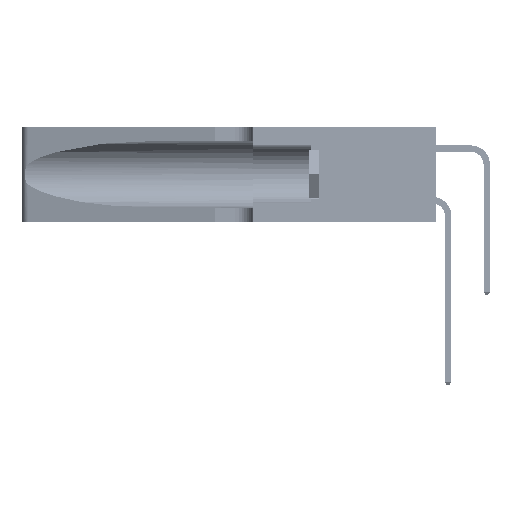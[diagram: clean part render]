
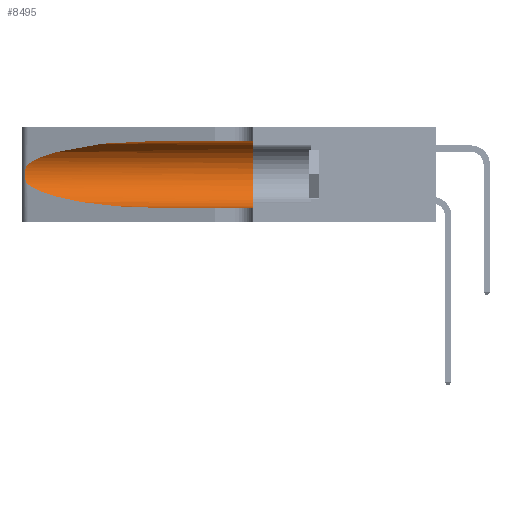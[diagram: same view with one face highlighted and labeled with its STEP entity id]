
A CAD part, left-side view. The second image highlights one B-rep face of the part: STEP entity #8495.
In plain terms, the highlighted cylindrical face has radius 3.308 mm (diameter 6.617 mm), a partial arc.
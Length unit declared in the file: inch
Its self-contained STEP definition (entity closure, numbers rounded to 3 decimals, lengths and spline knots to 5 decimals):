
#243 = EDGE_CURVE ( 'NONE', #27568, #1937, #8975, .T. ) ;
#575 = DIRECTION ( 'NONE',  ( 0., 1., 0. ) ) ;
#1230 = CARTESIAN_POINT ( 'NONE',  ( 0.25487, 1.22718, 0.14631 ) ) ;
#1275 = CARTESIAN_POINT ( 'NONE',  ( 0.26018, 1.23835, 0.19895 ) ) ;
#1579 = DIRECTION ( 'NONE',  ( 0., -1., 0. ) ) ;
#1937 = VERTEX_POINT ( 'NONE', #19312 ) ;
#4107 = EDGE_CURVE ( 'NONE', #7412, #6198, #24047, .T. ) ;
#5278 = CARTESIAN_POINT ( 'NONE',  ( 0.2373, 1.15595, 0.08982 ) ) ;
#5326 = CARTESIAN_POINT ( 'NONE',  ( 0.26075, 1.23896, 0.178 ) ) ;
#5626 = DIRECTION ( 'NONE',  ( 0., 0., -1. ) ) ;
#6198 = VERTEX_POINT ( 'NONE', #50195 ) ;
#6496 = EDGE_LOOP ( 'NONE', ( #50033, #46082, #17295, #17205, #7360, #41811 ) ) ;
#7360 = ORIENTED_EDGE ( 'NONE', *, *, #22067, .F. ) ;
#7412 = VERTEX_POINT ( 'NONE', #39130 ) ;
#8495 = ADVANCED_FACE ( 'NONE', ( #29424 ), #28203, .F. ) ;
#8975 =( BOUNDED_CURVE ( )  B_SPLINE_CURVE ( 3, ( #45975, #42132, #22733, #49862 ),
 .UNSPECIFIED., .F., .T. ) 
 B_SPLINE_CURVE_WITH_KNOTS ( ( 4, 4 ),
 ( 1.5708, 2.84003 ),
 .UNSPECIFIED. ) 
 CURVE ( )  GEOMETRIC_REPRESENTATION_ITEM ( )  RATIONAL_B_SPLINE_CURVE ( ( 1., 0.87, 0.87, 1. ) ) 
 REPRESENTATION_ITEM ( '' )  );
#9319 = CARTESIAN_POINT ( 'NONE',  ( 0.1305, 0.72297, 0.05475 ) ) ;
#9369 = CARTESIAN_POINT ( 'NONE',  ( 0.25856, 1.23593, 0.16098 ) ) ;
#10896 = VERTEX_POINT ( 'NONE', #24713 ) ;
#12718 = AXIS2_PLACEMENT_3D ( 'NONE', #24147, #575, #28016 ) ;
#13281 = CARTESIAN_POINT ( 'NONE',  ( 0.25639, 1.23186, 0.15144 ) ) ;
#14935 = CARTESIAN_POINT ( 'NONE',  ( 0.1305, 1.61858, 0.31525 ) ) ;
#17163 = CARTESIAN_POINT ( 'NONE',  ( 0.25487, 1.22718, 0.14631 ) ) ;
#17205 = ORIENTED_EDGE ( 'NONE', *, *, #4107, .T. ) ;
#17295 = ORIENTED_EDGE ( 'NONE', *, *, #40828, .T. ) ;
#19312 = CARTESIAN_POINT ( 'NONE',  ( 0.25487, 1.22718, 0.22369 ) ) ;
#19588 = B_SPLINE_CURVE_WITH_KNOTS ( 'NONE', 3,
 ( #40303, #44173, #20939, #48054, #24803, #1275, #28687, #5326, #32610, #9369, #36507, #13281, #40468, #17163 ),
 .UNSPECIFIED., .F., .F.,
 ( 4, 2, 2, 2, 2, 2, 4 ),
 ( 0., 0.00027, 0.00053, 0.00107, 0.0016, 0.00187, 0.00214 ),
 .UNSPECIFIED. ) ;
#20324 = CARTESIAN_POINT ( 'NONE',  ( 0.1305, 1.61858, 0.05475 ) ) ;
#20939 = CARTESIAN_POINT ( 'NONE',  ( 0.25639, 1.23184, 0.21858 ) ) ;
#21217 = CARTESIAN_POINT ( 'NONE',  ( 0.1305, 1.61858, 0.185 ) ) ;
#22067 = EDGE_CURVE ( 'NONE', #10896, #6198, #35866, .T. ) ;
#22733 = CARTESIAN_POINT ( 'NONE',  ( 0.2373, 1.15595, 0.28018 ) ) ;
#24047 = LINE ( 'NONE', #20324, #33134 ) ;
#24147 = CARTESIAN_POINT ( 'NONE',  ( 0.1305, 0.35, 0.185 ) ) ;
#24713 = CARTESIAN_POINT ( 'NONE',  ( 0.1305, 0.35, 0.31525 ) ) ;
#24803 = CARTESIAN_POINT ( 'NONE',  ( 0.25854, 1.2359, 0.20912 ) ) ;
#27568 = VERTEX_POINT ( 'NONE', #48504 ) ;
#28016 = DIRECTION ( 'NONE',  ( 0., 0., 1. ) ) ;
#28203 = CYLINDRICAL_SURFACE ( 'NONE', #32509, 0.13025 ) ;
#28687 = CARTESIAN_POINT ( 'NONE',  ( 0.26075, 1.23896, 0.19203 ) ) ;
#28864 = EDGE_CURVE ( 'NONE', #1937, #29435, #19588, .T. ) ;
#29385 = VECTOR ( 'NONE', #34627, 39.37008 ) ;
#29424 = FACE_OUTER_BOUND ( 'NONE', #6496, .T. ) ;
#29435 = VERTEX_POINT ( 'NONE', #50085 ) ;
#30047 = EDGE_CURVE ( 'NONE', #27568, #10896, #30609, .T. ) ;
#30609 = LINE ( 'NONE', #14935, #29385 ) ;
#32509 = AXIS2_PLACEMENT_3D ( 'NONE', #21217, #1579, #5626 ) ;
#32563 = CARTESIAN_POINT ( 'NONE',  ( 0.18966, 0.96281, 0.05475 ) ) ;
#32610 = CARTESIAN_POINT ( 'NONE',  ( 0.26017, 1.23833, 0.17102 ) ) ;
#33134 = VECTOR ( 'NONE', #43573, 39.37008 ) ;
#34627 = DIRECTION ( 'NONE',  ( 0., -1., 0. ) ) ;
#35866 = CIRCLE ( 'NONE', #12718, 0.13025 ) ;
#36507 = CARTESIAN_POINT ( 'NONE',  ( 0.25789, 1.23486, 0.15765 ) ) ;
#39130 = CARTESIAN_POINT ( 'NONE',  ( 0.1305, 0.72297, 0.05475 ) ) ;
#40303 = CARTESIAN_POINT ( 'NONE',  ( 0.25487, 1.22718, 0.22369 ) ) ;
#40468 = CARTESIAN_POINT ( 'NONE',  ( 0.25555, 1.22993, 0.14849 ) ) ;
#40828 = EDGE_CURVE ( 'NONE', #29435, #7412, #42943, .T. ) ;
#41811 = ORIENTED_EDGE ( 'NONE', *, *, #30047, .F. ) ;
#42132 = CARTESIAN_POINT ( 'NONE',  ( 0.18966, 0.96281, 0.31525 ) ) ;
#42943 =( BOUNDED_CURVE ( )  B_SPLINE_CURVE ( 3, ( #1230, #5278, #32563, #9319 ),
 .UNSPECIFIED., .F., .F. ) 
 B_SPLINE_CURVE_WITH_KNOTS ( ( 4, 4 ),
 ( 3.44316, 4.71239 ),
 .UNSPECIFIED. ) 
 CURVE ( )  GEOMETRIC_REPRESENTATION_ITEM ( )  RATIONAL_B_SPLINE_CURVE ( ( 1., 0.87, 0.87, 1. ) ) 
 REPRESENTATION_ITEM ( '' )  );
#43573 = DIRECTION ( 'NONE',  ( 0., -1., 0. ) ) ;
#44173 = CARTESIAN_POINT ( 'NONE',  ( 0.25555, 1.22994, 0.2215 ) ) ;
#45975 = CARTESIAN_POINT ( 'NONE',  ( 0.1305, 0.72297, 0.31525 ) ) ;
#46082 = ORIENTED_EDGE ( 'NONE', *, *, #28864, .T. ) ;
#48054 = CARTESIAN_POINT ( 'NONE',  ( 0.25787, 1.23484, 0.2124 ) ) ;
#48504 = CARTESIAN_POINT ( 'NONE',  ( 0.1305, 0.72297, 0.31525 ) ) ;
#49862 = CARTESIAN_POINT ( 'NONE',  ( 0.25487, 1.22718, 0.22369 ) ) ;
#50033 = ORIENTED_EDGE ( 'NONE', *, *, #243, .T. ) ;
#50085 = CARTESIAN_POINT ( 'NONE',  ( 0.25487, 1.22718, 0.14631 ) ) ;
#50195 = CARTESIAN_POINT ( 'NONE',  ( 0.1305, 0.35, 0.05475 ) ) ;
